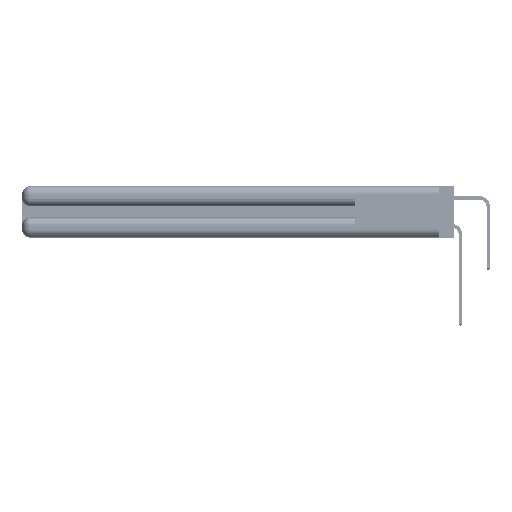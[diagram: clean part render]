
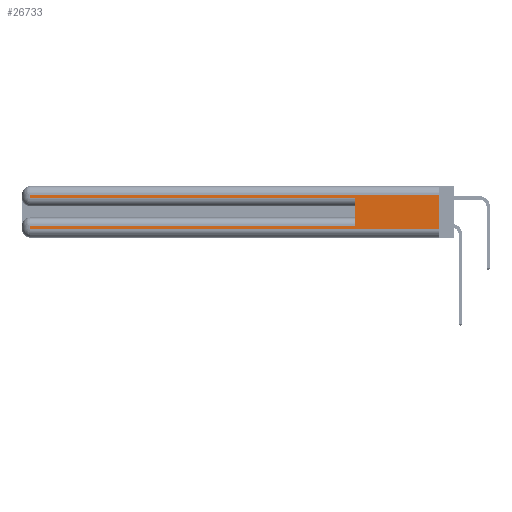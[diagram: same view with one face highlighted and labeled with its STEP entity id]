
A CAD part, left-side view. The second image highlights one B-rep face of the part: STEP entity #26733.
In plain terms, the highlighted planar face has unit normal (-1, 0, 0).
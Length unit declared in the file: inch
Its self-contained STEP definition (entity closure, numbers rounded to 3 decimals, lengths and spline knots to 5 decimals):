
#1344 = VERTEX_POINT ( 'NONE', #4829 ) ;
#1913 = LINE ( 'NONE', #8541, #44428 ) ;
#3457 = ORIENTED_EDGE ( 'NONE', *, *, #34114, .T. ) ;
#4210 = DIRECTION ( 'NONE',  ( 0., 0., -1. ) ) ;
#4567 = CARTESIAN_POINT ( 'NONE',  ( 0., 0., 0.285 ) ) ;
#4637 = DIRECTION ( 'NONE',  ( 0., 0., -1. ) ) ;
#4720 = VECTOR ( 'NONE', #8976, 39.37008 ) ;
#4829 = CARTESIAN_POINT ( 'NONE',  ( 0., 0.6, 0.285 ) ) ;
#6785 = ORIENTED_EDGE ( 'NONE', *, *, #15321, .T. ) ;
#7153 = VERTEX_POINT ( 'NONE', #15450 ) ;
#7799 = CARTESIAN_POINT ( 'NONE',  ( 0., 0., 0.085 ) ) ;
#7932 = VECTOR ( 'NONE', #22191, 39.37008 ) ;
#8541 = CARTESIAN_POINT ( 'NONE',  ( 0., 0., 0.06 ) ) ;
#8976 = DIRECTION ( 'NONE',  ( 0., 0., -1. ) ) ;
#11434 = ORIENTED_EDGE ( 'NONE', *, *, #36920, .F. ) ;
#11735 = EDGE_CURVE ( 'NONE', #33718, #1344, #30547, .T. ) ;
#12804 = DIRECTION ( 'NONE',  ( 0., -1., 0. ) ) ;
#13576 = CARTESIAN_POINT ( 'NONE',  ( 0., 2.94, 0.37 ) ) ;
#15321 = EDGE_CURVE ( 'NONE', #37686, #1344, #50556, .T. ) ;
#15450 = CARTESIAN_POINT ( 'NONE',  ( 0., 2.94, 0.085 ) ) ;
#15462 = VECTOR ( 'NONE', #51085, 39.37008 ) ;
#15979 = EDGE_CURVE ( 'NONE', #7153, #27847, #16056, .T. ) ;
#16056 = LINE ( 'NONE', #25909, #4720 ) ;
#16183 = FACE_OUTER_BOUND ( 'NONE', #34947, .T. ) ;
#16843 = CARTESIAN_POINT ( 'NONE',  ( 0., 0., 0.37 ) ) ;
#18625 = CARTESIAN_POINT ( 'NONE',  ( 0., 0.6, 0.085 ) ) ;
#19261 = LINE ( 'NONE', #38786, #51704 ) ;
#19704 = CARTESIAN_POINT ( 'NONE',  ( 0., 0., 0.06 ) ) ;
#20073 = VERTEX_POINT ( 'NONE', #51509 ) ;
#20738 = ORIENTED_EDGE ( 'NONE', *, *, #11735, .F. ) ;
#21056 = VERTEX_POINT ( 'NONE', #48016 ) ;
#21108 = DIRECTION ( 'NONE',  ( 1., 0., 0. ) ) ;
#22191 = DIRECTION ( 'NONE',  ( 0., 0., 1. ) ) ;
#24075 = ORIENTED_EDGE ( 'NONE', *, *, #28713, .T. ) ;
#25452 = CARTESIAN_POINT ( 'NONE',  ( 0., 0., 0.37 ) ) ;
#25487 = AXIS2_PLACEMENT_3D ( 'NONE', #16843, #21108, #50714 ) ;
#25909 = CARTESIAN_POINT ( 'NONE',  ( 0., 2.94, 0.37 ) ) ;
#26172 = EDGE_CURVE ( 'NONE', #20073, #37686, #53989, .T. ) ;
#26733 = ADVANCED_FACE ( 'NONE', ( #16183 ), #42265, .F. ) ;
#27847 = VERTEX_POINT ( 'NONE', #53968 ) ;
#28713 = EDGE_CURVE ( 'NONE', #21056, #20073, #19261, .T. ) ;
#30245 = DIRECTION ( 'NONE',  ( 0., 1., 0. ) ) ;
#30547 = LINE ( 'NONE', #43350, #7932 ) ;
#33718 = VERTEX_POINT ( 'NONE', #18625 ) ;
#33879 = VERTEX_POINT ( 'NONE', #19704 ) ;
#34114 = EDGE_CURVE ( 'NONE', #27847, #33879, #1913, .T. ) ;
#34736 = ORIENTED_EDGE ( 'NONE', *, *, #15979, .T. ) ;
#34947 = EDGE_LOOP ( 'NONE', ( #11434, #24075, #49234, #6785, #20738, #54514, #34736, #3457 ) ) ;
#36920 = EDGE_CURVE ( 'NONE', #21056, #33879, #38987, .T. ) ;
#37565 = VECTOR ( 'NONE', #50226, 39.37008 ) ;
#37656 = VECTOR ( 'NONE', #4210, 39.37008 ) ;
#37686 = VERTEX_POINT ( 'NONE', #51223 ) ;
#38786 = CARTESIAN_POINT ( 'NONE',  ( 0., 0., 0.31 ) ) ;
#38987 = LINE ( 'NONE', #25452, #37656 ) ;
#41492 = VECTOR ( 'NONE', #4637, 39.37008 ) ;
#42265 = PLANE ( 'NONE',  #25487 ) ;
#43350 = CARTESIAN_POINT ( 'NONE',  ( 0., 0.6, 0.145 ) ) ;
#44428 = VECTOR ( 'NONE', #12804, 39.37008 ) ;
#48016 = CARTESIAN_POINT ( 'NONE',  ( 0., 0., 0.31 ) ) ;
#48739 = LINE ( 'NONE', #7799, #37565 ) ;
#49234 = ORIENTED_EDGE ( 'NONE', *, *, #26172, .T. ) ;
#49721 = EDGE_CURVE ( 'NONE', #33718, #7153, #48739, .T. ) ;
#50226 = DIRECTION ( 'NONE',  ( 0., 1., 0. ) ) ;
#50556 = LINE ( 'NONE', #4567, #15462 ) ;
#50714 = DIRECTION ( 'NONE',  ( 0., 0., -1. ) ) ;
#51085 = DIRECTION ( 'NONE',  ( 0., -1., 0. ) ) ;
#51223 = CARTESIAN_POINT ( 'NONE',  ( 0., 2.94, 0.285 ) ) ;
#51509 = CARTESIAN_POINT ( 'NONE',  ( 0., 2.94, 0.31 ) ) ;
#51704 = VECTOR ( 'NONE', #30245, 39.37008 ) ;
#53968 = CARTESIAN_POINT ( 'NONE',  ( 0., 2.94, 0.06 ) ) ;
#53989 = LINE ( 'NONE', #13576, #41492 ) ;
#54514 = ORIENTED_EDGE ( 'NONE', *, *, #49721, .T. ) ;
